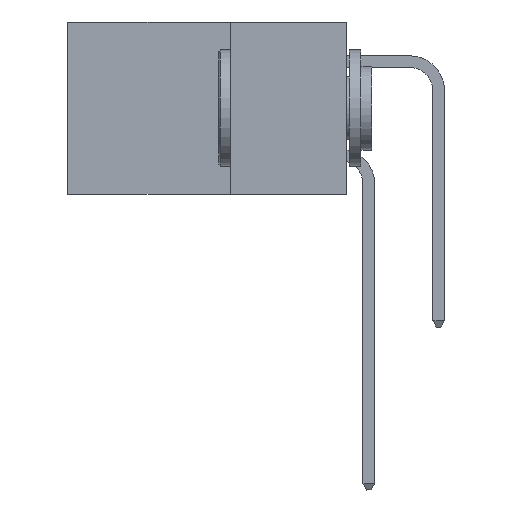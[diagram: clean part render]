
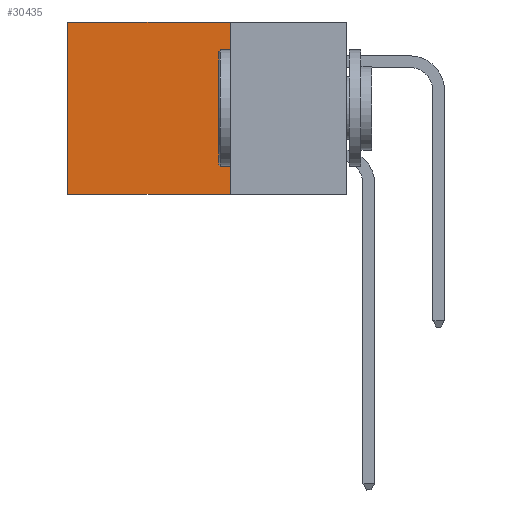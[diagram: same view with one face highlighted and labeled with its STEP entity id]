
A CAD part, left-side view. The second image highlights one B-rep face of the part: STEP entity #30435.
In plain terms, the highlighted planar face has unit normal (-1, 0, 0).
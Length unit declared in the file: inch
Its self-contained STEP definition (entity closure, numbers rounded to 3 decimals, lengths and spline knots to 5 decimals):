
#144 = ORIENTED_EDGE ( 'NONE', *, *, #29894, .F. ) ;
#967 = VERTEX_POINT ( 'NONE', #6538 ) ;
#3919 = VERTEX_POINT ( 'NONE', #31154 ) ;
#3924 = DIRECTION ( 'NONE',  ( 0., 1., 0. ) ) ;
#4897 = CARTESIAN_POINT ( 'NONE',  ( 0.2875, 0.6, 0. ) ) ;
#5106 = LINE ( 'NONE', #17766, #18472 ) ;
#5259 = EDGE_CURVE ( 'NONE', #27412, #3919, #34634, .T. ) ;
#5262 = ORIENTED_EDGE ( 'NONE', *, *, #31979, .T. ) ;
#5550 = DIRECTION ( 'NONE',  ( 0., 0., -1. ) ) ;
#6538 = CARTESIAN_POINT ( 'NONE',  ( 0.2875, 0.25, -0.37 ) ) ;
#7427 = ORIENTED_EDGE ( 'NONE', *, *, #15302, .F. ) ;
#8830 = CARTESIAN_POINT ( 'NONE',  ( 0.2875, 0.25, -0.37 ) ) ;
#11285 = VERTEX_POINT ( 'NONE', #32619 ) ;
#12878 = CARTESIAN_POINT ( 'NONE',  ( 0.2875, 0.25, 0. ) ) ;
#13252 = DIRECTION ( 'NONE',  ( 1., 0., 0. ) ) ;
#14180 = EDGE_LOOP ( 'NONE', ( #17492, #144, #7427, #5262 ) ) ;
#15302 = EDGE_CURVE ( 'NONE', #11285, #967, #5106, .T. ) ;
#15977 = CARTESIAN_POINT ( 'NONE',  ( 0.2875, 0.6, 0. ) ) ;
#17492 = ORIENTED_EDGE ( 'NONE', *, *, #5259, .T. ) ;
#17766 = CARTESIAN_POINT ( 'NONE',  ( 0.2875, 0.25, 0. ) ) ;
#18472 = VECTOR ( 'NONE', #26599, 39.37008 ) ;
#20916 = DIRECTION ( 'NONE',  ( 0., 1., 0. ) ) ;
#20942 = VECTOR ( 'NONE', #3924, 39.37008 ) ;
#23735 = VECTOR ( 'NONE', #20916, 39.37008 ) ;
#24246 = FACE_OUTER_BOUND ( 'NONE', #14180, .T. ) ;
#25114 = LINE ( 'NONE', #8830, #20942 ) ;
#26562 = CARTESIAN_POINT ( 'NONE',  ( 0.2875, 0.25, 0. ) ) ;
#26599 = DIRECTION ( 'NONE',  ( 0., 0., -1. ) ) ;
#27412 = VERTEX_POINT ( 'NONE', #4897 ) ;
#27497 = VECTOR ( 'NONE', #5550, 39.37008 ) ;
#29377 = PLANE ( 'NONE',  #30098 ) ;
#29894 = EDGE_CURVE ( 'NONE', #967, #3919, #25114, .T. ) ;
#30098 = AXIS2_PLACEMENT_3D ( 'NONE', #26562, #13252, #34637 ) ;
#30435 = ADVANCED_FACE ( 'NONE', ( #24246 ), #29377, .F. ) ;
#30862 = LINE ( 'NONE', #12878, #23735 ) ;
#31154 = CARTESIAN_POINT ( 'NONE',  ( 0.2875, 0.6, -0.37 ) ) ;
#31979 = EDGE_CURVE ( 'NONE', #11285, #27412, #30862, .T. ) ;
#32619 = CARTESIAN_POINT ( 'NONE',  ( 0.2875, 0.25, 0. ) ) ;
#34634 = LINE ( 'NONE', #15977, #27497 ) ;
#34637 = DIRECTION ( 'NONE',  ( 0., 0., -1. ) ) ;
